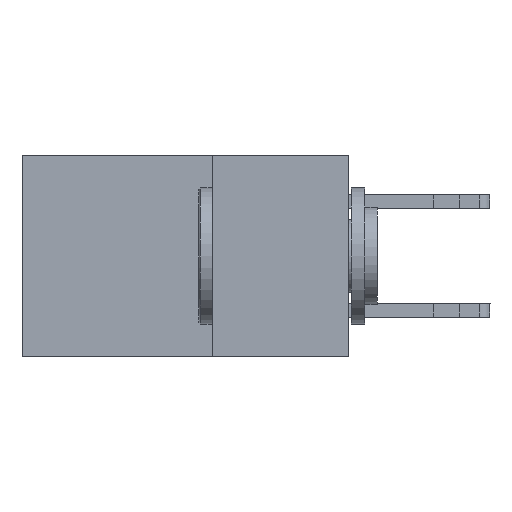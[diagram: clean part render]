
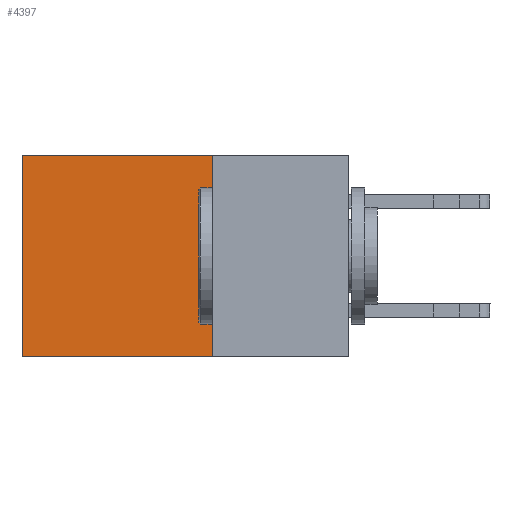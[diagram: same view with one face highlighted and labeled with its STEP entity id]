
A CAD part, left-side view. The second image highlights one B-rep face of the part: STEP entity #4397.
In plain terms, the highlighted planar face has unit normal (-1, 0, 0).
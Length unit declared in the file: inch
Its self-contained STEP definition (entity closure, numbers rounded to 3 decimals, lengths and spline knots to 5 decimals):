
#133 = CARTESIAN_POINT ( 'NONE',  ( 0.2615, 0.25, -0.37 ) ) ;
#390 = EDGE_CURVE ( 'NONE', #12051, #7824, #14155, .T. ) ;
#578 = ORIENTED_EDGE ( 'NONE', *, *, #16667, .F. ) ;
#900 = LINE ( 'NONE', #9883, #14046 ) ;
#1698 = VECTOR ( 'NONE', #2194, 39.37008 ) ;
#2050 = CARTESIAN_POINT ( 'NONE',  ( 0.2615, 0.6, -0.37 ) ) ;
#2194 = DIRECTION ( 'NONE',  ( 0., 1., 0. ) ) ;
#2739 = AXIS2_PLACEMENT_3D ( 'NONE', #12730, #12131, #12087 ) ;
#2988 = ORIENTED_EDGE ( 'NONE', *, *, #13323, .T. ) ;
#3165 = VERTEX_POINT ( 'NONE', #13840 ) ;
#4397 = ADVANCED_FACE ( 'NONE', ( #11275 ), #12936, .F. ) ;
#6047 = DIRECTION ( 'NONE',  ( 0., 1., 0. ) ) ;
#7824 = VERTEX_POINT ( 'NONE', #13572 ) ;
#8760 = LINE ( 'NONE', #11321, #1698 ) ;
#8848 = VECTOR ( 'NONE', #6047, 39.37008 ) ;
#9883 = CARTESIAN_POINT ( 'NONE',  ( 0.2615, 0.6, -0.37 ) ) ;
#11178 = ORIENTED_EDGE ( 'NONE', *, *, #390, .F. ) ;
#11192 = DIRECTION ( 'NONE',  ( 0., 0., -1. ) ) ;
#11275 = FACE_OUTER_BOUND ( 'NONE', #15333, .T. ) ;
#11321 = CARTESIAN_POINT ( 'NONE',  ( 0.2615, 0.25, 0. ) ) ;
#11392 = CARTESIAN_POINT ( 'NONE',  ( 0.2615, 0.25, 0. ) ) ;
#11663 = ORIENTED_EDGE ( 'NONE', *, *, #14988, .T. ) ;
#12051 = VERTEX_POINT ( 'NONE', #11392 ) ;
#12087 = DIRECTION ( 'NONE',  ( 0., 0., -1. ) ) ;
#12131 = DIRECTION ( 'NONE',  ( 1., 0., 0. ) ) ;
#12730 = CARTESIAN_POINT ( 'NONE',  ( 0.2615, 0.25, -0.37 ) ) ;
#12936 = PLANE ( 'NONE',  #2739 ) ;
#13323 = EDGE_CURVE ( 'NONE', #3165, #15545, #900, .T. ) ;
#13572 = CARTESIAN_POINT ( 'NONE',  ( 0.2615, 0.25, -0.37 ) ) ;
#13770 = VECTOR ( 'NONE', #15687, 39.37008 ) ;
#13840 = CARTESIAN_POINT ( 'NONE',  ( 0.2615, 0.6, 0. ) ) ;
#14046 = VECTOR ( 'NONE', #11192, 39.37008 ) ;
#14155 = LINE ( 'NONE', #133, #13770 ) ;
#14988 = EDGE_CURVE ( 'NONE', #12051, #3165, #8760, .T. ) ;
#15333 = EDGE_LOOP ( 'NONE', ( #2988, #578, #11178, #11663 ) ) ;
#15545 = VERTEX_POINT ( 'NONE', #2050 ) ;
#15610 = LINE ( 'NONE', #16268, #8848 ) ;
#15687 = DIRECTION ( 'NONE',  ( 0., 0., -1. ) ) ;
#16268 = CARTESIAN_POINT ( 'NONE',  ( 0.2615, 0.25, -0.37 ) ) ;
#16667 = EDGE_CURVE ( 'NONE', #7824, #15545, #15610, .T. ) ;
